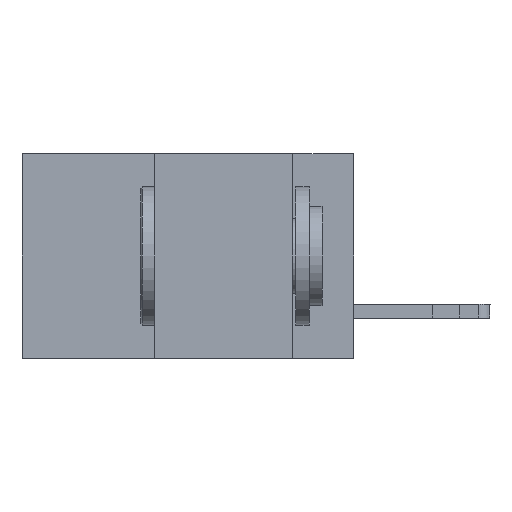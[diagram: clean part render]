
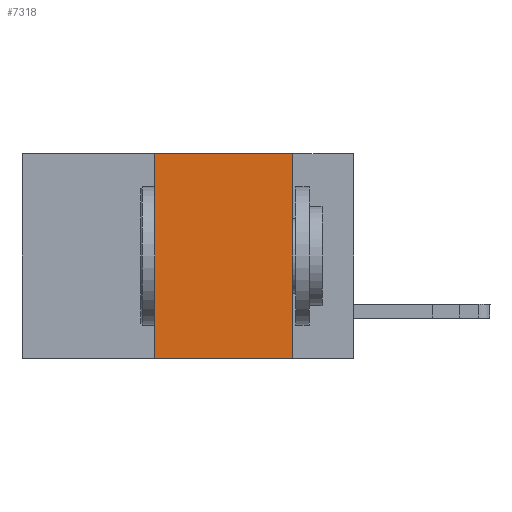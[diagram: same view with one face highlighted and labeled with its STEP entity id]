
A CAD part, left-side view. The second image highlights one B-rep face of the part: STEP entity #7318.
In plain terms, the highlighted planar face has unit normal (-1, 0, 0).
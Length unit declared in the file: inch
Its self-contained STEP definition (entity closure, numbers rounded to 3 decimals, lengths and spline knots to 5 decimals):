
#1262 = ORIENTED_EDGE ( 'NONE', *, *, #11760, .F. ) ;
#1797 = CARTESIAN_POINT ( 'NONE',  ( 0., 0.11, -0.37 ) ) ;
#2038 = LINE ( 'NONE', #11240, #10717 ) ;
#6994 = DIRECTION ( 'NONE',  ( 1., 0., 0. ) ) ;
#7318 = ADVANCED_FACE ( 'NONE', ( #11235 ), #13811, .F. ) ;
#8170 = CARTESIAN_POINT ( 'NONE',  ( 0., 0.6, 0. ) ) ;
#8824 = DIRECTION ( 'NONE',  ( 0., 0., -1. ) ) ;
#8906 = DIRECTION ( 'NONE',  ( 0., -1., 0. ) ) ;
#9416 = CARTESIAN_POINT ( 'NONE',  ( 0., 0.36, 0. ) ) ;
#10131 = VERTEX_POINT ( 'NONE', #17577 ) ;
#10717 = VECTOR ( 'NONE', #8824, 39.37008 ) ;
#11235 = FACE_OUTER_BOUND ( 'NONE', #25651, .T. ) ;
#11240 = CARTESIAN_POINT ( 'NONE',  ( 0., 0.11, 0. ) ) ;
#11760 = EDGE_CURVE ( 'NONE', #10131, #29410, #2038, .T. ) ;
#13177 = DIRECTION ( 'NONE',  ( 0., 0., 1. ) ) ;
#13803 = VECTOR ( 'NONE', #8906, 39.37008 ) ;
#13811 = PLANE ( 'NONE',  #16885 ) ;
#15135 = LINE ( 'NONE', #17400, #27299 ) ;
#15480 = EDGE_CURVE ( 'NONE', #26347, #27635, #15135, .T. ) ;
#15604 = DIRECTION ( 'NONE',  ( 0., -1., 0. ) ) ;
#15727 = EDGE_CURVE ( 'NONE', #26347, #29410, #20420, .T. ) ;
#16224 = DIRECTION ( 'NONE',  ( 0., 0., -1. ) ) ;
#16885 = AXIS2_PLACEMENT_3D ( 'NONE', #23018, #6994, #16224 ) ;
#17400 = CARTESIAN_POINT ( 'NONE',  ( 0., 0.36, 0. ) ) ;
#17577 = CARTESIAN_POINT ( 'NONE',  ( 0., 0.11, 0. ) ) ;
#18721 = ORIENTED_EDGE ( 'NONE', *, *, #15727, .T. ) ;
#20420 = LINE ( 'NONE', #29600, #13803 ) ;
#22413 = LINE ( 'NONE', #8170, #24349 ) ;
#23018 = CARTESIAN_POINT ( 'NONE',  ( 0., 0.6, 0. ) ) ;
#24154 = EDGE_CURVE ( 'NONE', #27635, #10131, #22413, .T. ) ;
#24349 = VECTOR ( 'NONE', #15604, 39.37008 ) ;
#25574 = ORIENTED_EDGE ( 'NONE', *, *, #24154, .F. ) ;
#25651 = EDGE_LOOP ( 'NONE', ( #1262, #25574, #27283, #18721 ) ) ;
#26347 = VERTEX_POINT ( 'NONE', #27287 ) ;
#27283 = ORIENTED_EDGE ( 'NONE', *, *, #15480, .F. ) ;
#27287 = CARTESIAN_POINT ( 'NONE',  ( 0., 0.36, -0.37 ) ) ;
#27299 = VECTOR ( 'NONE', #13177, 39.37008 ) ;
#27635 = VERTEX_POINT ( 'NONE', #9416 ) ;
#29410 = VERTEX_POINT ( 'NONE', #1797 ) ;
#29600 = CARTESIAN_POINT ( 'NONE',  ( 0., 0.6, -0.37 ) ) ;
